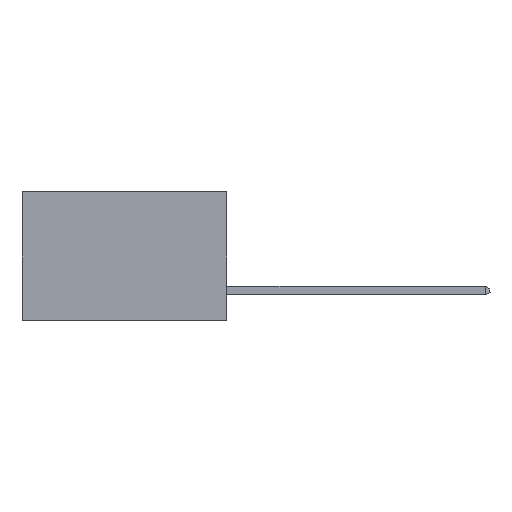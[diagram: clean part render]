
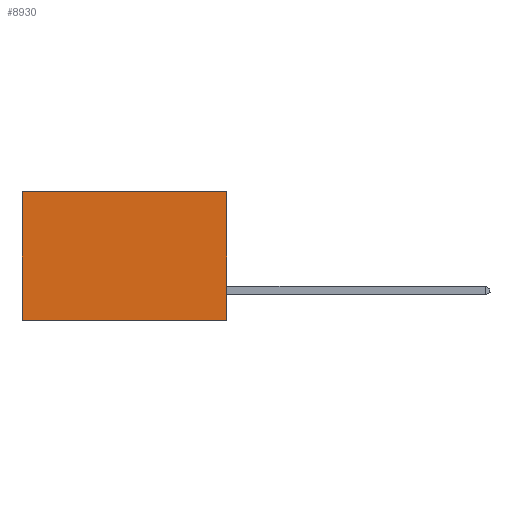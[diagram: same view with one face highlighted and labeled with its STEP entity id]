
A CAD part, left-side view. The second image highlights one B-rep face of the part: STEP entity #8930.
In plain terms, the highlighted planar face has unit normal (-1, 0, 0).
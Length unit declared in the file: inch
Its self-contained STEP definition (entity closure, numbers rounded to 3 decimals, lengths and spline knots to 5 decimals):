
#388 = LINE ( 'NONE', #4417, #5766 ) ;
#3027 = ORIENTED_EDGE ( 'NONE', *, *, #19731, .F. ) ;
#3151 = DIRECTION ( 'NONE',  ( 0., 0., -1. ) ) ;
#3523 = DIRECTION ( 'NONE',  ( 0., 1., 0. ) ) ;
#4417 = CARTESIAN_POINT ( 'NONE',  ( 0.277, 0.59, -0.37 ) ) ;
#5104 = FACE_OUTER_BOUND ( 'NONE', #24060, .T. ) ;
#5203 = LINE ( 'NONE', #15590, #9927 ) ;
#5523 = LINE ( 'NONE', #23199, #20303 ) ;
#5766 = VECTOR ( 'NONE', #12465, 39.37008 ) ;
#6091 = VERTEX_POINT ( 'NONE', #11979 ) ;
#7663 = DIRECTION ( 'NONE',  ( 0., 1., 0. ) ) ;
#7822 = ORIENTED_EDGE ( 'NONE', *, *, #16006, .T. ) ;
#8145 = LINE ( 'NONE', #19686, #24801 ) ;
#8930 = ADVANCED_FACE ( 'NONE', ( #5104 ), #20797, .F. ) ;
#9927 = VECTOR ( 'NONE', #3523, 39.37008 ) ;
#11352 = ORIENTED_EDGE ( 'NONE', *, *, #21236, .T. ) ;
#11979 = CARTESIAN_POINT ( 'NONE',  ( 0.277, 0.59, 0. ) ) ;
#12255 = CARTESIAN_POINT ( 'NONE',  ( 0.277, 0., 0. ) ) ;
#12465 = DIRECTION ( 'NONE',  ( 0., 0., -1. ) ) ;
#12780 = VERTEX_POINT ( 'NONE', #18649 ) ;
#15043 = CARTESIAN_POINT ( 'NONE',  ( 0.277, 0.59, -0.37 ) ) ;
#15590 = CARTESIAN_POINT ( 'NONE',  ( 0.277, 0., -0.37 ) ) ;
#15754 = AXIS2_PLACEMENT_3D ( 'NONE', #20702, #20587, #20556 ) ;
#16006 = EDGE_CURVE ( 'NONE', #19965, #6091, #8145, .T. ) ;
#16755 = ORIENTED_EDGE ( 'NONE', *, *, #20145, .F. ) ;
#18649 = CARTESIAN_POINT ( 'NONE',  ( 0.277, 0., -0.37 ) ) ;
#19686 = CARTESIAN_POINT ( 'NONE',  ( 0.277, 0., 0. ) ) ;
#19731 = EDGE_CURVE ( 'NONE', #12780, #24199, #5203, .T. ) ;
#19965 = VERTEX_POINT ( 'NONE', #12255 ) ;
#20145 = EDGE_CURVE ( 'NONE', #19965, #12780, #5523, .T. ) ;
#20303 = VECTOR ( 'NONE', #3151, 39.37008 ) ;
#20556 = DIRECTION ( 'NONE',  ( 0., 0., -1. ) ) ;
#20587 = DIRECTION ( 'NONE',  ( 1., 0., 0. ) ) ;
#20702 = CARTESIAN_POINT ( 'NONE',  ( 0.277, 0., -0.37 ) ) ;
#20797 = PLANE ( 'NONE',  #15754 ) ;
#21236 = EDGE_CURVE ( 'NONE', #6091, #24199, #388, .T. ) ;
#23199 = CARTESIAN_POINT ( 'NONE',  ( 0.277, 0., -0.37 ) ) ;
#24060 = EDGE_LOOP ( 'NONE', ( #11352, #3027, #16755, #7822 ) ) ;
#24199 = VERTEX_POINT ( 'NONE', #15043 ) ;
#24801 = VECTOR ( 'NONE', #7663, 39.37008 ) ;
